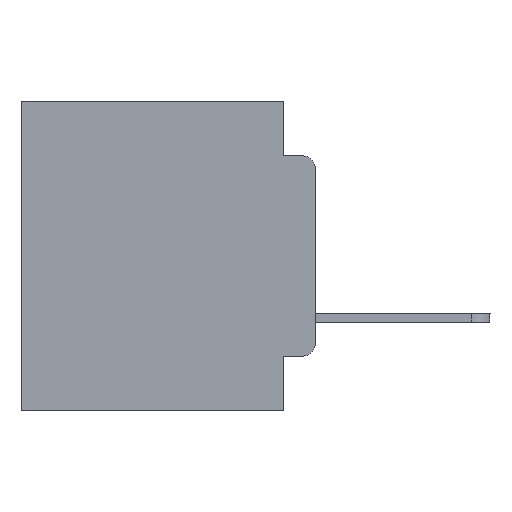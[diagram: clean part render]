
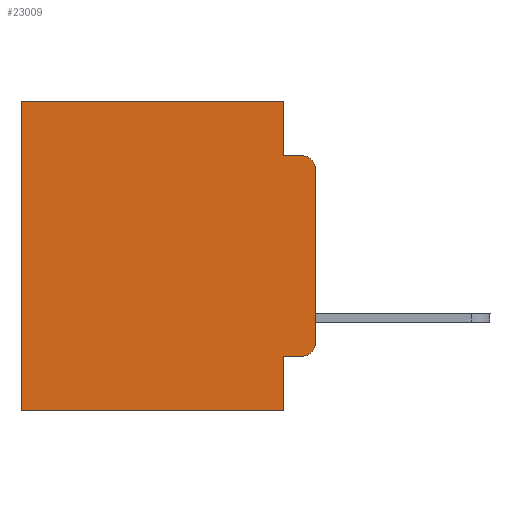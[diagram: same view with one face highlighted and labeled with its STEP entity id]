
A CAD part, left-side view. The second image highlights one B-rep face of the part: STEP entity #23009.
In plain terms, the highlighted planar face has unit normal (-1, 0, 0).
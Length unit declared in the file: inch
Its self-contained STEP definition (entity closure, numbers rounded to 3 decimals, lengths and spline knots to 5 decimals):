
#924 = EDGE_CURVE ( 'NONE', #12218, #2657, #13933, .T. ) ;
#960 = VERTEX_POINT ( 'NONE', #8093 ) ;
#1139 = ORIENTED_EDGE ( 'NONE', *, *, #23713, .T. ) ;
#2044 = CARTESIAN_POINT ( 'NONE',  ( 0.298, 0.02, -0.3915 ) ) ;
#2141 = VECTOR ( 'NONE', #4001, 39.37008 ) ;
#2338 = CARTESIAN_POINT ( 'NONE',  ( 0.298, 0.02, -0.0885 ) ) ;
#2657 = VERTEX_POINT ( 'NONE', #3714 ) ;
#3569 = DIRECTION ( 'NONE',  ( 0., -1., 0. ) ) ;
#3683 = ORIENTED_EDGE ( 'NONE', *, *, #24868, .F. ) ;
#3714 = CARTESIAN_POINT ( 'NONE',  ( 0.298, 0.051, -0.0885 ) ) ;
#3922 = VERTEX_POINT ( 'NONE', #13327 ) ;
#3948 = VECTOR ( 'NONE', #20754, 39.37008 ) ;
#4001 = DIRECTION ( 'NONE',  ( 0., 0., -1. ) ) ;
#4020 = AXIS2_PLACEMENT_3D ( 'NONE', #12619, #20766, #18743 ) ;
#4499 = AXIS2_PLACEMENT_3D ( 'NONE', #2044, #6144, #6000 ) ;
#5075 = CARTESIAN_POINT ( 'NONE',  ( 0.298, 0.051, 0. ) ) ;
#5385 = LINE ( 'NONE', #21970, #13479 ) ;
#5585 = EDGE_CURVE ( 'NONE', #3922, #15651, #12253, .T. ) ;
#5950 = VECTOR ( 'NONE', #10228, 39.37008 ) ;
#6000 = DIRECTION ( 'NONE',  ( 0., 0., -1. ) ) ;
#6144 = DIRECTION ( 'NONE',  ( -1., 0., 0. ) ) ;
#6437 = DIRECTION ( 'NONE',  ( 0., -1., 0. ) ) ;
#6564 = ORIENTED_EDGE ( 'NONE', *, *, #924, .F. ) ;
#6689 = ORIENTED_EDGE ( 'NONE', *, *, #21133, .T. ) ;
#7201 = VERTEX_POINT ( 'NONE', #11445 ) ;
#7640 = CARTESIAN_POINT ( 'NONE',  ( 0.298, 0.02, -0.1085 ) ) ;
#7660 = ORIENTED_EDGE ( 'NONE', *, *, #5585, .F. ) ;
#8093 = CARTESIAN_POINT ( 'NONE',  ( 0.298, 0.02, -0.4115 ) ) ;
#8491 = CARTESIAN_POINT ( 'NONE',  ( 0.298, 0.051, -0.0885 ) ) ;
#8742 = AXIS2_PLACEMENT_3D ( 'NONE', #7640, #12205, #26133 ) ;
#9851 = VECTOR ( 'NONE', #6437, 39.37008 ) ;
#9959 = VERTEX_POINT ( 'NONE', #2338 ) ;
#10030 = EDGE_CURVE ( 'NONE', #7201, #15651, #12533, .T. ) ;
#10228 = DIRECTION ( 'NONE',  ( 0., 1., 0. ) ) ;
#10272 = CARTESIAN_POINT ( 'NONE',  ( 0.298, 0., -0.3915 ) ) ;
#10477 = ORIENTED_EDGE ( 'NONE', *, *, #13881, .F. ) ;
#10764 = ORIENTED_EDGE ( 'NONE', *, *, #10030, .T. ) ;
#11335 = LINE ( 'NONE', #19756, #19341 ) ;
#11445 = CARTESIAN_POINT ( 'NONE',  ( 0.298, 0.473, 0. ) ) ;
#11465 = LINE ( 'NONE', #17711, #12738 ) ;
#11727 = DIRECTION ( 'NONE',  ( 0., 0., -1. ) ) ;
#12205 = DIRECTION ( 'NONE',  ( -1., 0., 0. ) ) ;
#12218 = VERTEX_POINT ( 'NONE', #5075 ) ;
#12253 = LINE ( 'NONE', #20539, #5950 ) ;
#12533 = LINE ( 'NONE', #25325, #25650 ) ;
#12619 = CARTESIAN_POINT ( 'NONE',  ( 0.298, 0., 0. ) ) ;
#12738 = VECTOR ( 'NONE', #3569, 39.37008 ) ;
#12810 = DIRECTION ( 'NONE',  ( 0., 0., -1. ) ) ;
#13183 = CIRCLE ( 'NONE', #4499, 0.02 ) ;
#13327 = CARTESIAN_POINT ( 'NONE',  ( 0.298, 0.051, -0.5 ) ) ;
#13360 = ORIENTED_EDGE ( 'NONE', *, *, #21037, .T. ) ;
#13479 = VECTOR ( 'NONE', #17621, 39.37008 ) ;
#13709 = ORIENTED_EDGE ( 'NONE', *, *, #14101, .F. ) ;
#13797 = CARTESIAN_POINT ( 'NONE',  ( 0.298, 0.051, 0. ) ) ;
#13881 = EDGE_CURVE ( 'NONE', #2657, #9959, #17035, .T. ) ;
#13921 = VERTEX_POINT ( 'NONE', #15008 ) ;
#13933 = LINE ( 'NONE', #13797, #2141 ) ;
#14101 = EDGE_CURVE ( 'NONE', #13921, #26190, #11335, .T. ) ;
#14522 = LINE ( 'NONE', #22809, #3948 ) ;
#14546 = ORIENTED_EDGE ( 'NONE', *, *, #23521, .T. ) ;
#14942 = FACE_OUTER_BOUND ( 'NONE', #21856, .T. ) ;
#15008 = CARTESIAN_POINT ( 'NONE',  ( 0.298, 0., -0.1085 ) ) ;
#15651 = VERTEX_POINT ( 'NONE', #23794 ) ;
#15840 = CARTESIAN_POINT ( 'NONE',  ( 0.298, 0.051, -0.4115 ) ) ;
#17035 = LINE ( 'NONE', #8491, #9851 ) ;
#17621 = DIRECTION ( 'NONE',  ( 0., 0., -1. ) ) ;
#17711 = CARTESIAN_POINT ( 'NONE',  ( 0.298, 0.051, -0.4115 ) ) ;
#18743 = DIRECTION ( 'NONE',  ( 0., 0., -1. ) ) ;
#18881 = PLANE ( 'NONE',  #4020 ) ;
#19341 = VECTOR ( 'NONE', #11727, 39.37008 ) ;
#19756 = CARTESIAN_POINT ( 'NONE',  ( 0.298, 0., 0. ) ) ;
#20539 = CARTESIAN_POINT ( 'NONE',  ( 0.298, 0., -0.5 ) ) ;
#20754 = DIRECTION ( 'NONE',  ( 0., 1., 0. ) ) ;
#20766 = DIRECTION ( 'NONE',  ( 1., 0., 0. ) ) ;
#21037 = EDGE_CURVE ( 'NONE', #13921, #9959, #22597, .T. ) ;
#21133 = EDGE_CURVE ( 'NONE', #12218, #7201, #14522, .T. ) ;
#21856 = EDGE_LOOP ( 'NONE', ( #13709, #13360, #10477, #6564, #6689, #10764, #7660, #3683, #14546, #1139 ) ) ;
#21970 = CARTESIAN_POINT ( 'NONE',  ( 0.298, 0.051, 0. ) ) ;
#22597 = CIRCLE ( 'NONE', #8742, 0.02 ) ;
#22809 = CARTESIAN_POINT ( 'NONE',  ( 0.298, 0., 0. ) ) ;
#23009 = ADVANCED_FACE ( 'NONE', ( #14942 ), #18881, .F. ) ;
#23111 = VERTEX_POINT ( 'NONE', #15840 ) ;
#23521 = EDGE_CURVE ( 'NONE', #23111, #960, #11465, .T. ) ;
#23713 = EDGE_CURVE ( 'NONE', #960, #26190, #13183, .T. ) ;
#23794 = CARTESIAN_POINT ( 'NONE',  ( 0.298, 0.473, -0.5 ) ) ;
#24868 = EDGE_CURVE ( 'NONE', #23111, #3922, #5385, .T. ) ;
#25325 = CARTESIAN_POINT ( 'NONE',  ( 0.298, 0.473, 0. ) ) ;
#25650 = VECTOR ( 'NONE', #12810, 39.37008 ) ;
#26133 = DIRECTION ( 'NONE',  ( 0., 0., -1. ) ) ;
#26190 = VERTEX_POINT ( 'NONE', #10272 ) ;
